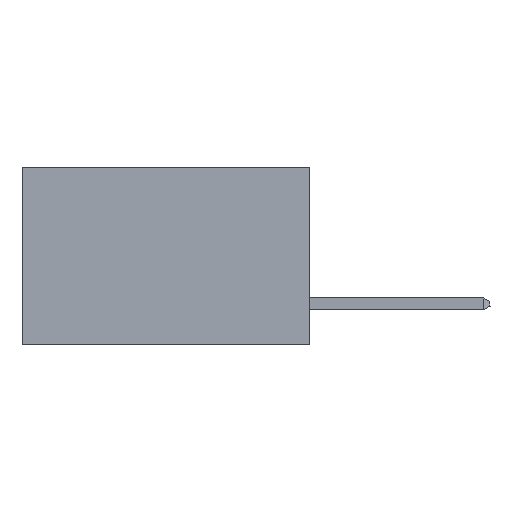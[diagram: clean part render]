
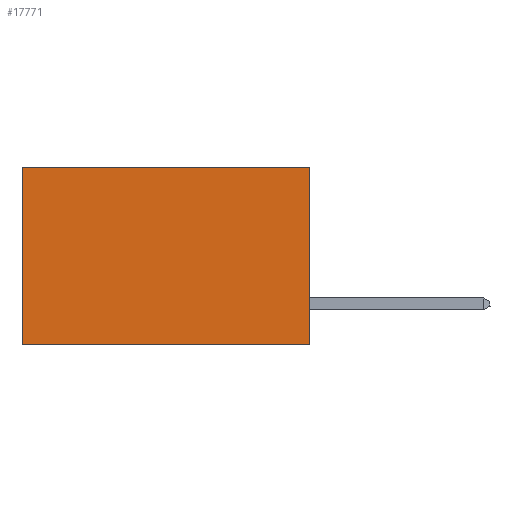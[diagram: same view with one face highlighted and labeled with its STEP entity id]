
A CAD part, left-side view. The second image highlights one B-rep face of the part: STEP entity #17771.
In plain terms, the highlighted planar face has unit normal (-1, 0, 0).
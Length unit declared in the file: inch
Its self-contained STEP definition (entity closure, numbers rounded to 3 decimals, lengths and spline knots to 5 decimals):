
#123 = CARTESIAN_POINT ( 'NONE',  ( 0.2875, 0.6, -0.37 ) ) ;
#1267 = CARTESIAN_POINT ( 'NONE',  ( 0.2875, 0.6, 0. ) ) ;
#2161 = ORIENTED_EDGE ( 'NONE', *, *, #24438, .T. ) ;
#2733 = EDGE_LOOP ( 'NONE', ( #2161, #34885, #26275, #8165 ) ) ;
#3812 = DIRECTION ( 'NONE',  ( 1., 0., 0. ) ) ;
#4568 = DIRECTION ( 'NONE',  ( 0., 1., 0. ) ) ;
#5292 = VECTOR ( 'NONE', #21576, 39.37008 ) ;
#7131 = DIRECTION ( 'NONE',  ( 0., 1., 0. ) ) ;
#8165 = ORIENTED_EDGE ( 'NONE', *, *, #30737, .T. ) ;
#8682 = LINE ( 'NONE', #16416, #38105 ) ;
#10199 = VECTOR ( 'NONE', #14027, 39.37008 ) ;
#10978 = CARTESIAN_POINT ( 'NONE',  ( 0.2875, 0., 0. ) ) ;
#14027 = DIRECTION ( 'NONE',  ( 0., 0., -1. ) ) ;
#15361 = FACE_OUTER_BOUND ( 'NONE', #2733, .T. ) ;
#16416 = CARTESIAN_POINT ( 'NONE',  ( 0.2875, 0., -0.37 ) ) ;
#17418 = VERTEX_POINT ( 'NONE', #1267 ) ;
#17771 = ADVANCED_FACE ( 'NONE', ( #15361 ), #21424, .F. ) ;
#19311 = VECTOR ( 'NONE', #7131, 39.37008 ) ;
#20937 = LINE ( 'NONE', #30294, #5292 ) ;
#21424 = PLANE ( 'NONE',  #38024 ) ;
#21576 = DIRECTION ( 'NONE',  ( 0., 0., -1. ) ) ;
#22117 = CARTESIAN_POINT ( 'NONE',  ( 0.2875, 0., -0.37 ) ) ;
#24362 = DIRECTION ( 'NONE',  ( 0., 0., -1. ) ) ;
#24438 = EDGE_CURVE ( 'NONE', #17418, #33956, #20937, .T. ) ;
#25235 = VERTEX_POINT ( 'NONE', #30897 ) ;
#26275 = ORIENTED_EDGE ( 'NONE', *, *, #37981, .F. ) ;
#26608 = CARTESIAN_POINT ( 'NONE',  ( 0.2875, 0., 0. ) ) ;
#28460 = VERTEX_POINT ( 'NONE', #22117 ) ;
#28479 = LINE ( 'NONE', #26608, #19311 ) ;
#28977 = LINE ( 'NONE', #10978, #10199 ) ;
#30294 = CARTESIAN_POINT ( 'NONE',  ( 0.2875, 0.6, 0. ) ) ;
#30737 = EDGE_CURVE ( 'NONE', #25235, #17418, #28479, .T. ) ;
#30897 = CARTESIAN_POINT ( 'NONE',  ( 0.2875, 0., 0. ) ) ;
#31524 = EDGE_CURVE ( 'NONE', #28460, #33956, #8682, .T. ) ;
#33956 = VERTEX_POINT ( 'NONE', #123 ) ;
#34885 = ORIENTED_EDGE ( 'NONE', *, *, #31524, .F. ) ;
#36229 = CARTESIAN_POINT ( 'NONE',  ( 0.2875, 0., 0. ) ) ;
#37981 = EDGE_CURVE ( 'NONE', #25235, #28460, #28977, .T. ) ;
#38024 = AXIS2_PLACEMENT_3D ( 'NONE', #36229, #3812, #24362 ) ;
#38105 = VECTOR ( 'NONE', #4568, 39.37008 ) ;
